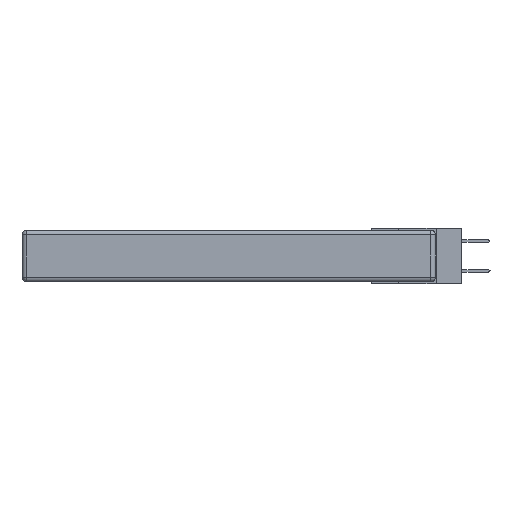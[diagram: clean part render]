
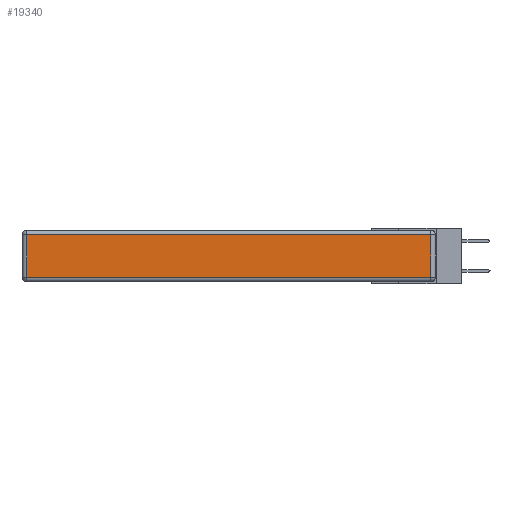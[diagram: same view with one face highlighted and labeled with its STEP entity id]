
A CAD part, left-side view. The second image highlights one B-rep face of the part: STEP entity #19340.
In plain terms, the highlighted planar face has unit normal (-1, 0, 0).
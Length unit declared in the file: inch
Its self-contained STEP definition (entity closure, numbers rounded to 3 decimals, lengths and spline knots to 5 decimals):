
#311 = LINE ( 'NONE', #8244, #21073 ) ;
#630 = ORIENTED_EDGE ( 'NONE', *, *, #19846, .T. ) ;
#2651 = ORIENTED_EDGE ( 'NONE', *, *, #2890, .T. ) ;
#2890 = EDGE_CURVE ( 'NONE', #3572, #12213, #14384, .T. ) ;
#3250 = VECTOR ( 'NONE', #12084, 39.37008 ) ;
#3572 = VERTEX_POINT ( 'NONE', #22033 ) ;
#4043 = EDGE_LOOP ( 'NONE', ( #25167, #20437, #2651, #630 ) ) ;
#4059 = DIRECTION ( 'NONE',  ( 0., 0., 1. ) ) ;
#4912 = DIRECTION ( 'NONE',  ( -1., 0., 0. ) ) ;
#6780 = CARTESIAN_POINT ( 'NONE',  ( 0., 2.72, -0.03 ) ) ;
#7162 = CARTESIAN_POINT ( 'NONE',  ( 0., 0., -0.313 ) ) ;
#8244 = CARTESIAN_POINT ( 'NONE',  ( 0., 2.72, -0.343 ) ) ;
#9010 = CARTESIAN_POINT ( 'NONE',  ( 0., 0.03, -0.313 ) ) ;
#12084 = DIRECTION ( 'NONE',  ( 0., -1., 0. ) ) ;
#12213 = VERTEX_POINT ( 'NONE', #6780 ) ;
#12511 = LINE ( 'NONE', #18529, #27885 ) ;
#14384 = LINE ( 'NONE', #23323, #30068 ) ;
#14456 = CARTESIAN_POINT ( 'NONE',  ( 0., 0., -0.343 ) ) ;
#14673 = DIRECTION ( 'NONE',  ( 0., 0., 1. ) ) ;
#15930 = VERTEX_POINT ( 'NONE', #21003 ) ;
#17019 = PLANE ( 'NONE',  #19799 ) ;
#17072 = LINE ( 'NONE', #7162, #3250 ) ;
#18529 = CARTESIAN_POINT ( 'NONE',  ( 0., 0.03, -0.343 ) ) ;
#18856 = EDGE_CURVE ( 'NONE', #15930, #20066, #17072, .T. ) ;
#19340 = ADVANCED_FACE ( 'NONE', ( #24712 ), #17019, .T. ) ;
#19799 = AXIS2_PLACEMENT_3D ( 'NONE', #14456, #4912, #14673 ) ;
#19846 = EDGE_CURVE ( 'NONE', #12213, #15930, #311, .T. ) ;
#20066 = VERTEX_POINT ( 'NONE', #9010 ) ;
#20316 = DIRECTION ( 'NONE',  ( 0., 0., -1. ) ) ;
#20437 = ORIENTED_EDGE ( 'NONE', *, *, #20628, .T. ) ;
#20628 = EDGE_CURVE ( 'NONE', #20066, #3572, #12511, .T. ) ;
#21003 = CARTESIAN_POINT ( 'NONE',  ( 0., 2.72, -0.313 ) ) ;
#21073 = VECTOR ( 'NONE', #20316, 39.37008 ) ;
#22033 = CARTESIAN_POINT ( 'NONE',  ( 0., 0.03, -0.03 ) ) ;
#23323 = CARTESIAN_POINT ( 'NONE',  ( 0., 2.75, -0.03 ) ) ;
#24712 = FACE_OUTER_BOUND ( 'NONE', #4043, .T. ) ;
#25167 = ORIENTED_EDGE ( 'NONE', *, *, #18856, .T. ) ;
#27885 = VECTOR ( 'NONE', #4059, 39.37008 ) ;
#30068 = VECTOR ( 'NONE', #30568, 39.37008 ) ;
#30568 = DIRECTION ( 'NONE',  ( 0., 1., 0. ) ) ;
